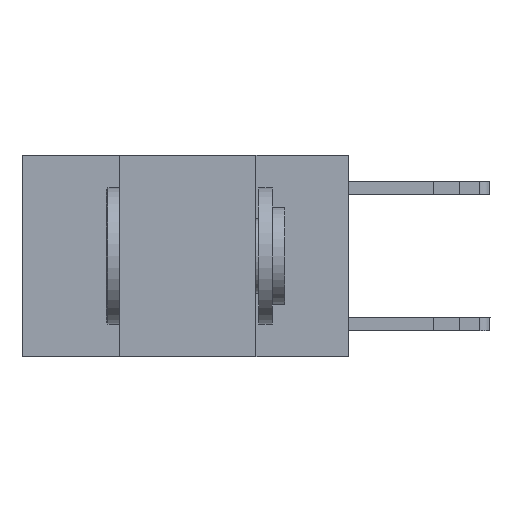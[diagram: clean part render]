
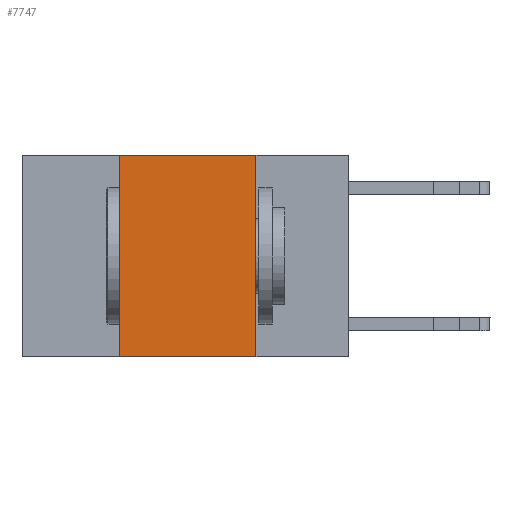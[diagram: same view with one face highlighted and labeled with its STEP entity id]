
A CAD part, left-side view. The second image highlights one B-rep face of the part: STEP entity #7747.
In plain terms, the highlighted planar face has unit normal (-1, 0, 0).
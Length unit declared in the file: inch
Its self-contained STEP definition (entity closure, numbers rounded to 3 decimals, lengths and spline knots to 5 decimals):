
#212 = DIRECTION ( 'NONE',  ( 0., 0., -1. ) ) ;
#501 = CARTESIAN_POINT ( 'NONE',  ( 0., 0.42, 0. ) ) ;
#685 = DIRECTION ( 'NONE',  ( 0., 0., 1. ) ) ;
#1070 = EDGE_CURVE ( 'NONE', #12618, #13857, #15610, .T. ) ;
#1431 = ORIENTED_EDGE ( 'NONE', *, *, #14097, .F. ) ;
#1457 = CARTESIAN_POINT ( 'NONE',  ( 0., 0.6, 0. ) ) ;
#1587 = CARTESIAN_POINT ( 'NONE',  ( 0., 0.17, -0.37 ) ) ;
#1713 = DIRECTION ( 'NONE',  ( 1., 0., 0. ) ) ;
#1899 = CARTESIAN_POINT ( 'NONE',  ( 0., 0.42, 0. ) ) ;
#1916 = VECTOR ( 'NONE', #15381, 39.37008 ) ;
#2013 = CARTESIAN_POINT ( 'NONE',  ( 0., 0.6, -0.37 ) ) ;
#2394 = ORIENTED_EDGE ( 'NONE', *, *, #1070, .F. ) ;
#3232 = VERTEX_POINT ( 'NONE', #14689 ) ;
#3733 = VERTEX_POINT ( 'NONE', #501 ) ;
#3767 = CARTESIAN_POINT ( 'NONE',  ( 0., 0.17, 0. ) ) ;
#5488 = FACE_OUTER_BOUND ( 'NONE', #13891, .T. ) ;
#5881 = VECTOR ( 'NONE', #9060, 39.37008 ) ;
#6098 = DIRECTION ( 'NONE',  ( 0., -1., 0. ) ) ;
#6255 = AXIS2_PLACEMENT_3D ( 'NONE', #1457, #1713, #212 ) ;
#7414 = LINE ( 'NONE', #12677, #7492 ) ;
#7492 = VECTOR ( 'NONE', #6098, 39.37008 ) ;
#7747 = ADVANCED_FACE ( 'NONE', ( #5488 ), #9487, .F. ) ;
#8880 = CARTESIAN_POINT ( 'NONE',  ( 0., 0.17, 0. ) ) ;
#8893 = ORIENTED_EDGE ( 'NONE', *, *, #15713, .F. ) ;
#9060 = DIRECTION ( 'NONE',  ( 0., 0., -1. ) ) ;
#9487 = PLANE ( 'NONE',  #6255 ) ;
#9744 = VECTOR ( 'NONE', #685, 39.37008 ) ;
#11413 = LINE ( 'NONE', #1899, #9744 ) ;
#12615 = LINE ( 'NONE', #2013, #1916 ) ;
#12618 = VERTEX_POINT ( 'NONE', #8880 ) ;
#12677 = CARTESIAN_POINT ( 'NONE',  ( 0., 0.6, 0. ) ) ;
#13857 = VERTEX_POINT ( 'NONE', #1587 ) ;
#13891 = EDGE_LOOP ( 'NONE', ( #2394, #1431, #8893, #15816 ) ) ;
#14097 = EDGE_CURVE ( 'NONE', #3733, #12618, #7414, .T. ) ;
#14689 = CARTESIAN_POINT ( 'NONE',  ( 0., 0.42, -0.37 ) ) ;
#15310 = EDGE_CURVE ( 'NONE', #3232, #13857, #12615, .T. ) ;
#15381 = DIRECTION ( 'NONE',  ( 0., -1., 0. ) ) ;
#15610 = LINE ( 'NONE', #3767, #5881 ) ;
#15713 = EDGE_CURVE ( 'NONE', #3232, #3733, #11413, .T. ) ;
#15816 = ORIENTED_EDGE ( 'NONE', *, *, #15310, .T. ) ;
